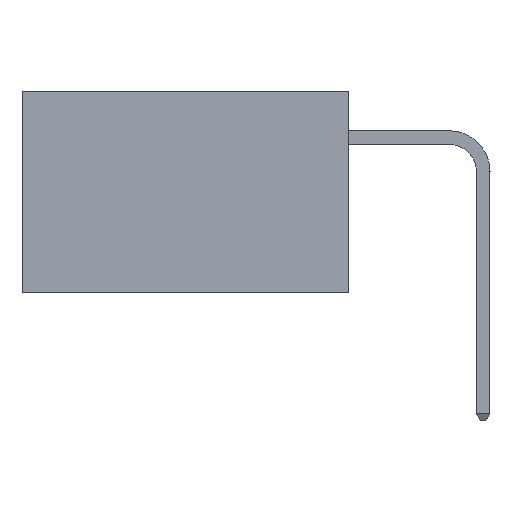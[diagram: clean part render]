
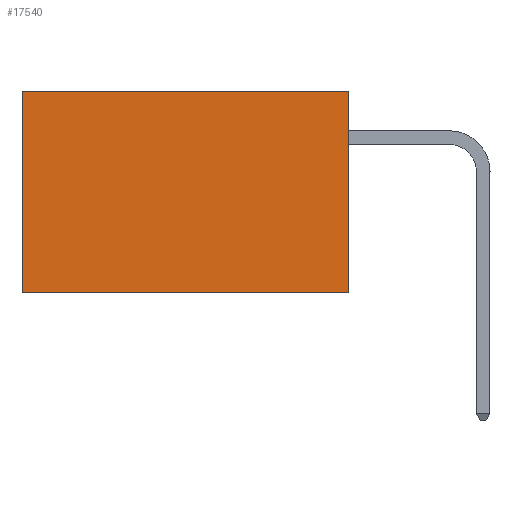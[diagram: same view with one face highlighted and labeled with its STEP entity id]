
A CAD part, left-side view. The second image highlights one B-rep face of the part: STEP entity #17540.
In plain terms, the highlighted planar face has unit normal (-1, 0, 0).
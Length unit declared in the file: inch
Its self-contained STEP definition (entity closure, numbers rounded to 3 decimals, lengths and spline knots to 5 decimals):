
#722 = LINE ( 'NONE', #5030, #28115 ) ;
#1049 = CARTESIAN_POINT ( 'NONE',  ( 0.2875, 0.6, 0. ) ) ;
#1062 = ORIENTED_EDGE ( 'NONE', *, *, #31531, .F. ) ;
#2533 = CARTESIAN_POINT ( 'NONE',  ( 0.2875, 0., -0.37 ) ) ;
#2666 = ORIENTED_EDGE ( 'NONE', *, *, #17403, .T. ) ;
#5030 = CARTESIAN_POINT ( 'NONE',  ( 0.2875, 0.6, 0. ) ) ;
#5560 = EDGE_CURVE ( 'NONE', #12012, #13883, #5821, .T. ) ;
#5821 = LINE ( 'NONE', #23815, #6618 ) ;
#6150 = ORIENTED_EDGE ( 'NONE', *, *, #5560, .T. ) ;
#6515 = ORIENTED_EDGE ( 'NONE', *, *, #13572, .F. ) ;
#6618 = VECTOR ( 'NONE', #31500, 39.37008 ) ;
#9812 = FACE_OUTER_BOUND ( 'NONE', #22561, .T. ) ;
#12012 = VERTEX_POINT ( 'NONE', #24590 ) ;
#12909 = LINE ( 'NONE', #15628, #19644 ) ;
#13572 = EDGE_CURVE ( 'NONE', #12012, #28875, #12909, .T. ) ;
#13883 = VERTEX_POINT ( 'NONE', #1049 ) ;
#14451 = AXIS2_PLACEMENT_3D ( 'NONE', #18379, #28501, #23455 ) ;
#15628 = CARTESIAN_POINT ( 'NONE',  ( 0.2875, 0., 0. ) ) ;
#16571 = VERTEX_POINT ( 'NONE', #25529 ) ;
#17403 = EDGE_CURVE ( 'NONE', #13883, #16571, #722, .T. ) ;
#17540 = ADVANCED_FACE ( 'NONE', ( #9812 ), #20920, .F. ) ;
#17854 = DIRECTION ( 'NONE',  ( 0., 0., -1. ) ) ;
#18257 = LINE ( 'NONE', #2533, #24195 ) ;
#18379 = CARTESIAN_POINT ( 'NONE',  ( 0.2875, 0., 0. ) ) ;
#19587 = CARTESIAN_POINT ( 'NONE',  ( 0.2875, 0., -0.37 ) ) ;
#19644 = VECTOR ( 'NONE', #30880, 39.37008 ) ;
#20537 = DIRECTION ( 'NONE',  ( 0., 1., 0. ) ) ;
#20920 = PLANE ( 'NONE',  #14451 ) ;
#22561 = EDGE_LOOP ( 'NONE', ( #2666, #1062, #6515, #6150 ) ) ;
#23455 = DIRECTION ( 'NONE',  ( 0., 0., -1. ) ) ;
#23815 = CARTESIAN_POINT ( 'NONE',  ( 0.2875, 0., 0. ) ) ;
#24195 = VECTOR ( 'NONE', #20537, 39.37008 ) ;
#24590 = CARTESIAN_POINT ( 'NONE',  ( 0.2875, 0., 0. ) ) ;
#25529 = CARTESIAN_POINT ( 'NONE',  ( 0.2875, 0.6, -0.37 ) ) ;
#28115 = VECTOR ( 'NONE', #17854, 39.37008 ) ;
#28501 = DIRECTION ( 'NONE',  ( 1., 0., 0. ) ) ;
#28875 = VERTEX_POINT ( 'NONE', #19587 ) ;
#30880 = DIRECTION ( 'NONE',  ( 0., 0., -1. ) ) ;
#31500 = DIRECTION ( 'NONE',  ( 0., 1., 0. ) ) ;
#31531 = EDGE_CURVE ( 'NONE', #28875, #16571, #18257, .T. ) ;
